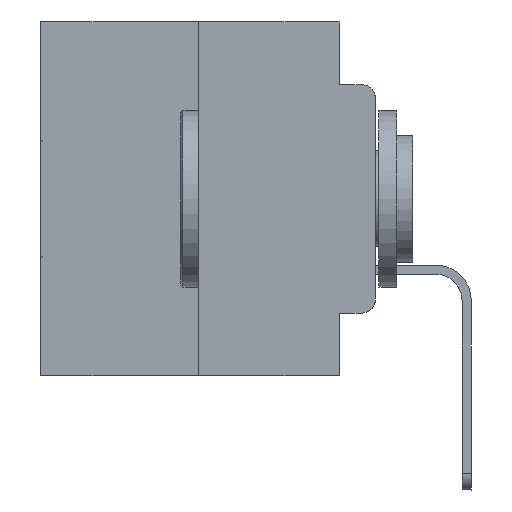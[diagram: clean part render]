
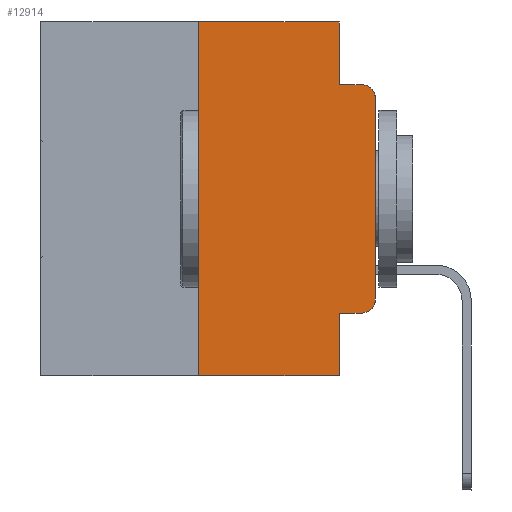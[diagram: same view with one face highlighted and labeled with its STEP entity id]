
A CAD part, left-side view. The second image highlights one B-rep face of the part: STEP entity #12914.
In plain terms, the highlighted planar face has unit normal (-1, 0, 0).
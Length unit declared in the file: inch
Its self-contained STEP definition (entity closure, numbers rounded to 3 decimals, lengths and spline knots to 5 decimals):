
#548 = CARTESIAN_POINT ( 'NONE',  ( 0., 0.02, -0.4115 ) ) ;
#616 = VERTEX_POINT ( 'NONE', #548 ) ;
#806 = AXIS2_PLACEMENT_3D ( 'NONE', #24265, #26556, #24359 ) ;
#1165 = EDGE_LOOP ( 'NONE', ( #10451, #13036, #9554, #1562, #19923, #23125, #7026, #18781, #18754, #19773 ) ) ;
#1562 = ORIENTED_EDGE ( 'NONE', *, *, #2140, .F. ) ;
#1798 = CARTESIAN_POINT ( 'NONE',  ( 0., 0., -0.1085 ) ) ;
#2140 = EDGE_CURVE ( 'NONE', #22030, #15517, #23325, .T. ) ;
#2474 = AXIS2_PLACEMENT_3D ( 'NONE', #12018, #28144, #7584 ) ;
#3276 = VECTOR ( 'NONE', #10401, 39.37008 ) ;
#4331 = VECTOR ( 'NONE', #23794, 39.37008 ) ;
#4486 = CARTESIAN_POINT ( 'NONE',  ( 0., 0.051, -0.4115 ) ) ;
#4708 = CARTESIAN_POINT ( 'NONE',  ( 0., 0.25, -0.5 ) ) ;
#5229 = DIRECTION ( 'NONE',  ( 0., -1., 0. ) ) ;
#5566 = LINE ( 'NONE', #23975, #13830 ) ;
#5786 = CARTESIAN_POINT ( 'NONE',  ( 0., 0., 0. ) ) ;
#5798 = CIRCLE ( 'NONE', #806, 0.02 ) ;
#6080 = CARTESIAN_POINT ( 'NONE',  ( 0., 0.051, -0.4115 ) ) ;
#6797 = EDGE_CURVE ( 'NONE', #15769, #28470, #21647, .T. ) ;
#7026 = ORIENTED_EDGE ( 'NONE', *, *, #11827, .T. ) ;
#7132 = LINE ( 'NONE', #17697, #8559 ) ;
#7329 = EDGE_CURVE ( 'NONE', #12156, #19976, #16191, .T. ) ;
#7584 = DIRECTION ( 'NONE',  ( 0., 0., -1. ) ) ;
#8559 = VECTOR ( 'NONE', #15665, 39.37008 ) ;
#8806 = VECTOR ( 'NONE', #17733, 39.37008 ) ;
#9196 = CARTESIAN_POINT ( 'NONE',  ( 0., 0.051, 0. ) ) ;
#9554 = ORIENTED_EDGE ( 'NONE', *, *, #13653, .F. ) ;
#10401 = DIRECTION ( 'NONE',  ( 0., 0., 1. ) ) ;
#10451 = ORIENTED_EDGE ( 'NONE', *, *, #6797, .T. ) ;
#10764 = EDGE_CURVE ( 'NONE', #12156, #616, #20358, .T. ) ;
#11827 = EDGE_CURVE ( 'NONE', #21395, #19976, #22989, .T. ) ;
#12018 = CARTESIAN_POINT ( 'NONE',  ( 0., 0.02, -0.1085 ) ) ;
#12156 = VERTEX_POINT ( 'NONE', #4486 ) ;
#12271 = DIRECTION ( 'NONE',  ( 0., 0., 1. ) ) ;
#12457 = DIRECTION ( 'NONE',  ( 0., -1., 0. ) ) ;
#12914 = ADVANCED_FACE ( 'NONE', ( #23641 ), #27609, .F. ) ;
#13036 = ORIENTED_EDGE ( 'NONE', *, *, #29428, .T. ) ;
#13653 = EDGE_CURVE ( 'NONE', #15517, #19766, #5566, .T. ) ;
#13779 = DIRECTION ( 'NONE',  ( 1., 0., 0. ) ) ;
#13830 = VECTOR ( 'NONE', #12457, 39.37008 ) ;
#15517 = VERTEX_POINT ( 'NONE', #17416 ) ;
#15630 = CARTESIAN_POINT ( 'NONE',  ( 0., 0.051, 0. ) ) ;
#15665 = DIRECTION ( 'NONE',  ( 0., -1., 0. ) ) ;
#15754 = VECTOR ( 'NONE', #5229, 39.37008 ) ;
#15769 = VERTEX_POINT ( 'NONE', #20851 ) ;
#15969 = CARTESIAN_POINT ( 'NONE',  ( 0., 0.25, 0. ) ) ;
#16191 = LINE ( 'NONE', #28500, #4331 ) ;
#16674 = CARTESIAN_POINT ( 'NONE',  ( 0., 0.051, -0.5 ) ) ;
#17186 = CARTESIAN_POINT ( 'NONE',  ( 0., 0.473, -0.5 ) ) ;
#17416 = CARTESIAN_POINT ( 'NONE',  ( 0., 0.051, -0.0885 ) ) ;
#17663 = DIRECTION ( 'NONE',  ( 0., 0., -1. ) ) ;
#17697 = CARTESIAN_POINT ( 'NONE',  ( 0., 0.473, 0. ) ) ;
#17733 = DIRECTION ( 'NONE',  ( 0., -1., 0. ) ) ;
#18754 = ORIENTED_EDGE ( 'NONE', *, *, #10764, .T. ) ;
#18781 = ORIENTED_EDGE ( 'NONE', *, *, #7329, .F. ) ;
#19341 = VECTOR ( 'NONE', #17663, 39.37008 ) ;
#19766 = VERTEX_POINT ( 'NONE', #29587 ) ;
#19773 = ORIENTED_EDGE ( 'NONE', *, *, #21769, .T. ) ;
#19923 = ORIENTED_EDGE ( 'NONE', *, *, #28482, .F. ) ;
#19976 = VERTEX_POINT ( 'NONE', #16674 ) ;
#20060 = CIRCLE ( 'NONE', #2474, 0.02 ) ;
#20358 = LINE ( 'NONE', #6080, #8806 ) ;
#20851 = CARTESIAN_POINT ( 'NONE',  ( 0., 0., -0.3915 ) ) ;
#21284 = VERTEX_POINT ( 'NONE', #15969 ) ;
#21395 = VERTEX_POINT ( 'NONE', #4708 ) ;
#21647 = LINE ( 'NONE', #5786, #3276 ) ;
#21769 = EDGE_CURVE ( 'NONE', #616, #15769, #5798, .T. ) ;
#22030 = VERTEX_POINT ( 'NONE', #9196 ) ;
#22309 = VECTOR ( 'NONE', #12271, 39.37008 ) ;
#22989 = LINE ( 'NONE', #17186, #15754 ) ;
#23125 = ORIENTED_EDGE ( 'NONE', *, *, #28346, .F. ) ;
#23325 = LINE ( 'NONE', #15630, #19341 ) ;
#23579 = CARTESIAN_POINT ( 'NONE',  ( 0., 0.25, 0. ) ) ;
#23641 = FACE_OUTER_BOUND ( 'NONE', #1165, .T. ) ;
#23794 = DIRECTION ( 'NONE',  ( 0., 0., -1. ) ) ;
#23975 = CARTESIAN_POINT ( 'NONE',  ( 0., 0.051, -0.0885 ) ) ;
#24265 = CARTESIAN_POINT ( 'NONE',  ( 0., 0.02, -0.3915 ) ) ;
#24359 = DIRECTION ( 'NONE',  ( 0., 0., -1. ) ) ;
#26556 = DIRECTION ( 'NONE',  ( -1., 0., 0. ) ) ;
#27609 = PLANE ( 'NONE',  #28952 ) ;
#28144 = DIRECTION ( 'NONE',  ( -1., 0., 0. ) ) ;
#28346 = EDGE_CURVE ( 'NONE', #21395, #21284, #29136, .T. ) ;
#28470 = VERTEX_POINT ( 'NONE', #1798 ) ;
#28482 = EDGE_CURVE ( 'NONE', #21284, #22030, #7132, .T. ) ;
#28500 = CARTESIAN_POINT ( 'NONE',  ( 0., 0.051, 0. ) ) ;
#28952 = AXIS2_PLACEMENT_3D ( 'NONE', #29720, #13779, #29811 ) ;
#29136 = LINE ( 'NONE', #23579, #22309 ) ;
#29428 = EDGE_CURVE ( 'NONE', #28470, #19766, #20060, .T. ) ;
#29587 = CARTESIAN_POINT ( 'NONE',  ( 0., 0.02, -0.0885 ) ) ;
#29720 = CARTESIAN_POINT ( 'NONE',  ( 0., 0.473, 0. ) ) ;
#29811 = DIRECTION ( 'NONE',  ( 0., 0., -1. ) ) ;
